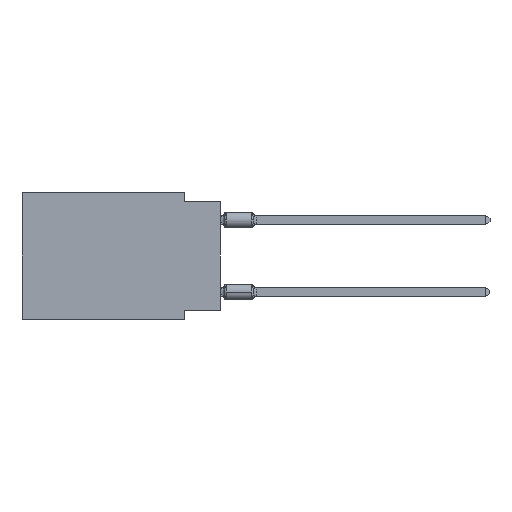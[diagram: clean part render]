
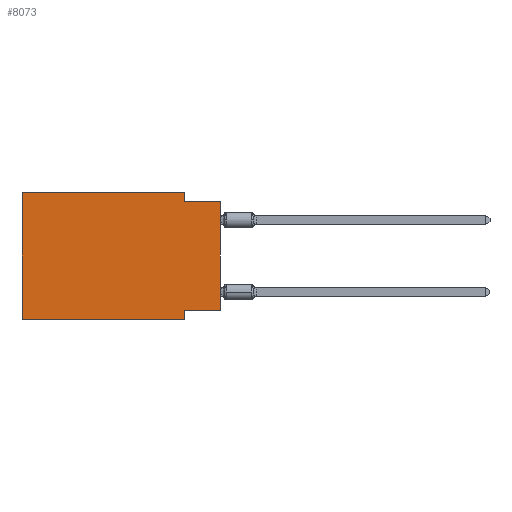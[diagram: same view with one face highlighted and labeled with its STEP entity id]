
A CAD part, left-side view. The second image highlights one B-rep face of the part: STEP entity #8073.
In plain terms, the highlighted planar face has unit normal (-1, 0, 0).
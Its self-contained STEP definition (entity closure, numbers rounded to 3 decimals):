
#274 = ORIENTED_EDGE ( 'NONE', *, *, #15051, .T. ) ;
#335 = CARTESIAN_POINT ( 'NONE',  ( 0., 13.97, -8.89 ) ) ;
#413 = AXIS2_PLACEMENT_3D ( 'NONE', #11350, #2270, #9837 ) ;
#454 = EDGE_CURVE ( 'NONE', #7956, #7649, #3734, .T. ) ;
#857 = CARTESIAN_POINT ( 'NONE',  ( 0., 13.97, -8.89 ) ) ;
#934 = EDGE_CURVE ( 'NONE', #19172, #19885, #20341, .T. ) ;
#1277 = LINE ( 'NONE', #19204, #18516 ) ;
#2270 = DIRECTION ( 'NONE',  ( 1., 0., 0. ) ) ;
#2641 = DIRECTION ( 'NONE',  ( 0., -1., 0. ) ) ;
#3676 = ORIENTED_EDGE ( 'NONE', *, *, #5094, .F. ) ;
#3734 = LINE ( 'NONE', #11398, #5185 ) ;
#3759 = EDGE_LOOP ( 'NONE', ( #13388, #13372, #3676, #14137, #6242, #274, #22190, #19869 ) ) ;
#3871 = VECTOR ( 'NONE', #15931, 1000. ) ;
#4765 = CARTESIAN_POINT ( 'NONE',  ( 0., 2.54, -8.255 ) ) ;
#4915 = EDGE_CURVE ( 'NONE', #10543, #7649, #21348, .T. ) ;
#5094 = EDGE_CURVE ( 'NONE', #12494, #10543, #1277, .T. ) ;
#5185 = VECTOR ( 'NONE', #20367, 1000. ) ;
#5222 = VECTOR ( 'NONE', #2641, 1000. ) ;
#5870 = CARTESIAN_POINT ( 'NONE',  ( 0., 2.54, 0. ) ) ;
#6242 = ORIENTED_EDGE ( 'NONE', *, *, #21118, .F. ) ;
#6414 = CARTESIAN_POINT ( 'NONE',  ( 0., 0., -0.635 ) ) ;
#7649 = VERTEX_POINT ( 'NONE', #6414 ) ;
#7956 = VERTEX_POINT ( 'NONE', #19627 ) ;
#8005 = LINE ( 'NONE', #20121, #5222 ) ;
#8048 = VERTEX_POINT ( 'NONE', #857 ) ;
#8073 = ADVANCED_FACE ( 'NONE', ( #15062 ), #13325, .F. ) ;
#8114 = VECTOR ( 'NONE', #17949, 1000. ) ;
#9507 = DIRECTION ( 'NONE',  ( 0., 0., 1. ) ) ;
#9837 = DIRECTION ( 'NONE',  ( 0., 0., -1. ) ) ;
#10221 = CARTESIAN_POINT ( 'NONE',  ( 0., 2.54, -0.635 ) ) ;
#10543 = VERTEX_POINT ( 'NONE', #10221 ) ;
#10821 = LINE ( 'NONE', #17921, #3871 ) ;
#11350 = CARTESIAN_POINT ( 'NONE',  ( 0., 13.97, 0. ) ) ;
#11398 = CARTESIAN_POINT ( 'NONE',  ( 0., 0., 0. ) ) ;
#12494 = VERTEX_POINT ( 'NONE', #5870 ) ;
#13325 = PLANE ( 'NONE',  #413 ) ;
#13372 = ORIENTED_EDGE ( 'NONE', *, *, #4915, .F. ) ;
#13388 = ORIENTED_EDGE ( 'NONE', *, *, #454, .T. ) ;
#13724 = DIRECTION ( 'NONE',  ( 0., 0., -1. ) ) ;
#14137 = ORIENTED_EDGE ( 'NONE', *, *, #16771, .F. ) ;
#14426 = VECTOR ( 'NONE', #22329, 1000. ) ;
#15051 = EDGE_CURVE ( 'NONE', #8048, #19885, #17361, .T. ) ;
#15062 = FACE_OUTER_BOUND ( 'NONE', #3759, .T. ) ;
#15323 = CARTESIAN_POINT ( 'NONE',  ( 0., 2.54, -8.89 ) ) ;
#15931 = DIRECTION ( 'NONE',  ( 0., 1., 0. ) ) ;
#16771 = EDGE_CURVE ( 'NONE', #18267, #12494, #8005, .T. ) ;
#17149 = CARTESIAN_POINT ( 'NONE',  ( 0., 2.54, -8.89 ) ) ;
#17361 = LINE ( 'NONE', #335, #21564 ) ;
#17721 = CARTESIAN_POINT ( 'NONE',  ( 0., 0., -0.635 ) ) ;
#17921 = CARTESIAN_POINT ( 'NONE',  ( 0., 0., -8.255 ) ) ;
#17949 = DIRECTION ( 'NONE',  ( 0., -1., 0. ) ) ;
#18267 = VERTEX_POINT ( 'NONE', #19979 ) ;
#18516 = VECTOR ( 'NONE', #13724, 1000. ) ;
#19172 = VERTEX_POINT ( 'NONE', #4765 ) ;
#19204 = CARTESIAN_POINT ( 'NONE',  ( 0., 2.54, 0. ) ) ;
#19319 = EDGE_CURVE ( 'NONE', #7956, #19172, #10821, .T. ) ;
#19627 = CARTESIAN_POINT ( 'NONE',  ( 0., 0., -8.255 ) ) ;
#19763 = LINE ( 'NONE', #19879, #21997 ) ;
#19869 = ORIENTED_EDGE ( 'NONE', *, *, #19319, .F. ) ;
#19879 = CARTESIAN_POINT ( 'NONE',  ( 0., 13.97, 0. ) ) ;
#19885 = VERTEX_POINT ( 'NONE', #17149 ) ;
#19979 = CARTESIAN_POINT ( 'NONE',  ( 0., 13.97, 0. ) ) ;
#20121 = CARTESIAN_POINT ( 'NONE',  ( 0., 13.97, 0. ) ) ;
#20341 = LINE ( 'NONE', #15323, #14426 ) ;
#20367 = DIRECTION ( 'NONE',  ( 0., 0., 1. ) ) ;
#21118 = EDGE_CURVE ( 'NONE', #8048, #18267, #19763, .T. ) ;
#21348 = LINE ( 'NONE', #17721, #8114 ) ;
#21561 = DIRECTION ( 'NONE',  ( 0., -1., 0. ) ) ;
#21564 = VECTOR ( 'NONE', #21561, 1000. ) ;
#21997 = VECTOR ( 'NONE', #9507, 1000. ) ;
#22190 = ORIENTED_EDGE ( 'NONE', *, *, #934, .F. ) ;
#22329 = DIRECTION ( 'NONE',  ( 0., 0., -1. ) ) ;
